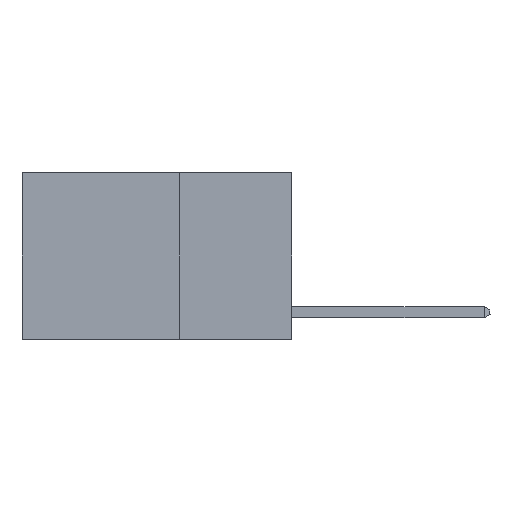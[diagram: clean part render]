
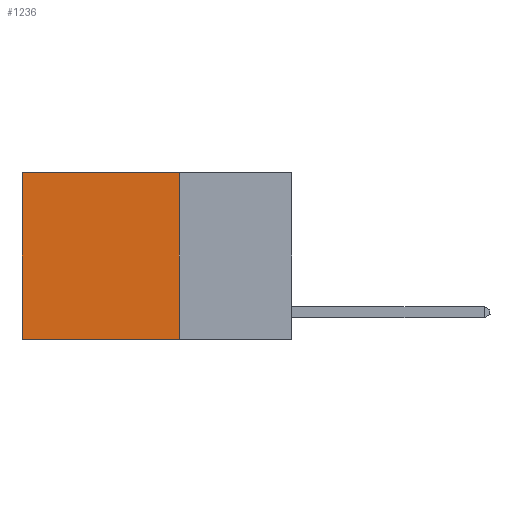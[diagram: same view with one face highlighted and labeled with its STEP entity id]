
A CAD part, left-side view. The second image highlights one B-rep face of the part: STEP entity #1236.
In plain terms, the highlighted planar face has unit normal (-1, 0, 0).
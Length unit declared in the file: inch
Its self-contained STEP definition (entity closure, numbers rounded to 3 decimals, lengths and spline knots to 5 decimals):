
#10 = DIRECTION ( 'NONE',  ( 0., 1., 0. ) ) ;
#63 = EDGE_CURVE ( 'NONE', #7129, #842, #6084, .T. ) ;
#599 = CARTESIAN_POINT ( 'NONE',  ( 0.2625, 0.25, 0. ) ) ;
#631 = CARTESIAN_POINT ( 'NONE',  ( 0.2625, 0.6, 0. ) ) ;
#842 = VERTEX_POINT ( 'NONE', #2598 ) ;
#1236 = ADVANCED_FACE ( 'NONE', ( #7702 ), #7556, .F. ) ;
#1258 = VERTEX_POINT ( 'NONE', #5504 ) ;
#1330 = CARTESIAN_POINT ( 'NONE',  ( 0.2625, 0.25, 0. ) ) ;
#1422 = DIRECTION ( 'NONE',  ( 0., 0., -1. ) ) ;
#2040 = DIRECTION ( 'NONE',  ( 1., 0., 0. ) ) ;
#2158 = ORIENTED_EDGE ( 'NONE', *, *, #4835, .F. ) ;
#2401 = LINE ( 'NONE', #7336, #4907 ) ;
#2598 = CARTESIAN_POINT ( 'NONE',  ( 0.2625, 0.6, -0.37 ) ) ;
#2701 = VECTOR ( 'NONE', #1422, 39.37008 ) ;
#3100 = AXIS2_PLACEMENT_3D ( 'NONE', #599, #2040, #3382 ) ;
#3308 = CARTESIAN_POINT ( 'NONE',  ( 0.2625, 0.25, -0.37 ) ) ;
#3382 = DIRECTION ( 'NONE',  ( 0., 0., -1. ) ) ;
#3846 = DIRECTION ( 'NONE',  ( 0., 1., 0. ) ) ;
#4030 = DIRECTION ( 'NONE',  ( 0., 0., -1. ) ) ;
#4298 = LINE ( 'NONE', #6328, #4618 ) ;
#4319 = ORIENTED_EDGE ( 'NONE', *, *, #63, .T. ) ;
#4618 = VECTOR ( 'NONE', #10, 39.37008 ) ;
#4717 = VECTOR ( 'NONE', #4030, 39.37008 ) ;
#4835 = EDGE_CURVE ( 'NONE', #1258, #5193, #7657, .T. ) ;
#4907 = VECTOR ( 'NONE', #3846, 39.37008 ) ;
#5193 = VERTEX_POINT ( 'NONE', #3308 ) ;
#5276 = ORIENTED_EDGE ( 'NONE', *, *, #7201, .T. ) ;
#5504 = CARTESIAN_POINT ( 'NONE',  ( 0.2625, 0.25, 0. ) ) ;
#6084 = LINE ( 'NONE', #8202, #4717 ) ;
#6328 = CARTESIAN_POINT ( 'NONE',  ( 0.2625, 0.25, -0.37 ) ) ;
#6390 = EDGE_LOOP ( 'NONE', ( #4319, #8180, #2158, #5276 ) ) ;
#7121 = EDGE_CURVE ( 'NONE', #5193, #842, #4298, .T. ) ;
#7129 = VERTEX_POINT ( 'NONE', #631 ) ;
#7201 = EDGE_CURVE ( 'NONE', #1258, #7129, #2401, .T. ) ;
#7336 = CARTESIAN_POINT ( 'NONE',  ( 0.2625, 0.25, 0. ) ) ;
#7556 = PLANE ( 'NONE',  #3100 ) ;
#7657 = LINE ( 'NONE', #1330, #2701 ) ;
#7702 = FACE_OUTER_BOUND ( 'NONE', #6390, .T. ) ;
#8180 = ORIENTED_EDGE ( 'NONE', *, *, #7121, .F. ) ;
#8202 = CARTESIAN_POINT ( 'NONE',  ( 0.2625, 0.6, 0. ) ) ;
